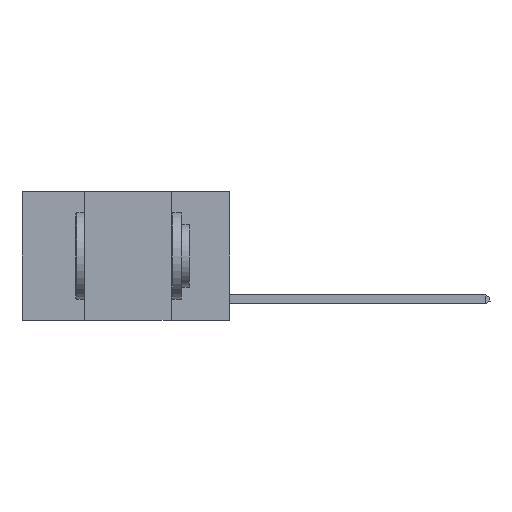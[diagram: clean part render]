
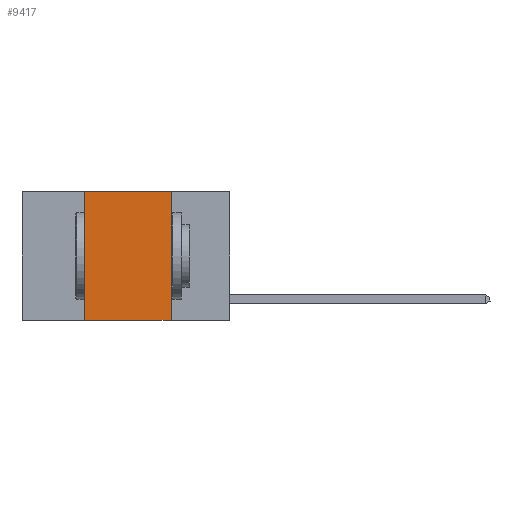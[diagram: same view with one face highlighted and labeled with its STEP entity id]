
A CAD part, left-side view. The second image highlights one B-rep face of the part: STEP entity #9417.
In plain terms, the highlighted planar face has unit normal (-1, 0, 0).
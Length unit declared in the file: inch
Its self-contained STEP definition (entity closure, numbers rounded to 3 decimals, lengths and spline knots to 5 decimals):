
#774 = DIRECTION ( 'NONE',  ( 0., 0., 1. ) ) ;
#1080 = CARTESIAN_POINT ( 'NONE',  ( 0., 0.17, -0.37 ) ) ;
#1561 = ORIENTED_EDGE ( 'NONE', *, *, #7842, .F. ) ;
#3321 = CARTESIAN_POINT ( 'NONE',  ( 0., 0.17, 0. ) ) ;
#3705 = AXIS2_PLACEMENT_3D ( 'NONE', #9253, #11317, #24385 ) ;
#3833 = VECTOR ( 'NONE', #11633, 39.37008 ) ;
#3947 = VERTEX_POINT ( 'NONE', #13439 ) ;
#4524 = EDGE_CURVE ( 'NONE', #18184, #8425, #7406, .T. ) ;
#5057 = LINE ( 'NONE', #9644, #3833 ) ;
#5155 = EDGE_CURVE ( 'NONE', #3947, #22586, #7069, .T. ) ;
#5377 = PLANE ( 'NONE',  #3705 ) ;
#6327 = CARTESIAN_POINT ( 'NONE',  ( 0., 0.6, -0.37 ) ) ;
#6495 = EDGE_CURVE ( 'NONE', #3947, #18184, #12538, .T. ) ;
#7069 = LINE ( 'NONE', #6327, #16727 ) ;
#7305 = VECTOR ( 'NONE', #774, 39.37008 ) ;
#7406 = LINE ( 'NONE', #19245, #17048 ) ;
#7842 = EDGE_CURVE ( 'NONE', #8425, #22586, #5057, .T. ) ;
#8425 = VERTEX_POINT ( 'NONE', #3321 ) ;
#9253 = CARTESIAN_POINT ( 'NONE',  ( 0., 0.6, 0. ) ) ;
#9417 = ADVANCED_FACE ( 'NONE', ( #17658 ), #5377, .F. ) ;
#9644 = CARTESIAN_POINT ( 'NONE',  ( 0., 0.17, 0. ) ) ;
#10289 = ORIENTED_EDGE ( 'NONE', *, *, #4524, .F. ) ;
#10296 = DIRECTION ( 'NONE',  ( 0., -1., 0. ) ) ;
#11317 = DIRECTION ( 'NONE',  ( 1., 0., 0. ) ) ;
#11633 = DIRECTION ( 'NONE',  ( 0., 0., -1. ) ) ;
#12362 = ORIENTED_EDGE ( 'NONE', *, *, #6495, .F. ) ;
#12538 = LINE ( 'NONE', #18256, #7305 ) ;
#13439 = CARTESIAN_POINT ( 'NONE',  ( 0., 0.42, -0.37 ) ) ;
#15481 = EDGE_LOOP ( 'NONE', ( #1561, #10289, #12362, #20279 ) ) ;
#16727 = VECTOR ( 'NONE', #10296, 39.37008 ) ;
#17048 = VECTOR ( 'NONE', #21130, 39.37008 ) ;
#17658 = FACE_OUTER_BOUND ( 'NONE', #15481, .T. ) ;
#18184 = VERTEX_POINT ( 'NONE', #22472 ) ;
#18256 = CARTESIAN_POINT ( 'NONE',  ( 0., 0.42, 0. ) ) ;
#19245 = CARTESIAN_POINT ( 'NONE',  ( 0., 0.6, 0. ) ) ;
#20279 = ORIENTED_EDGE ( 'NONE', *, *, #5155, .T. ) ;
#21130 = DIRECTION ( 'NONE',  ( 0., -1., 0. ) ) ;
#22472 = CARTESIAN_POINT ( 'NONE',  ( 0., 0.42, 0. ) ) ;
#22586 = VERTEX_POINT ( 'NONE', #1080 ) ;
#24385 = DIRECTION ( 'NONE',  ( 0., 0., -1. ) ) ;
